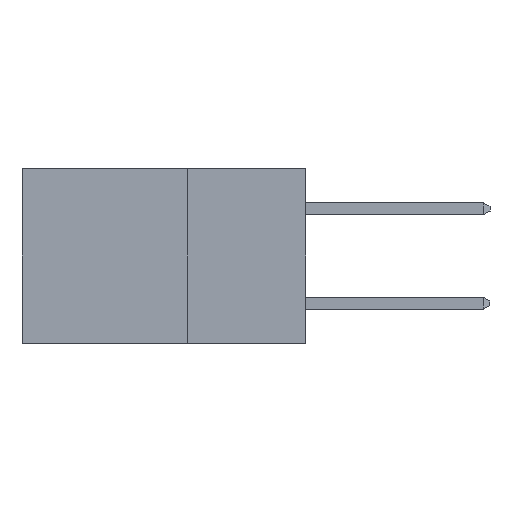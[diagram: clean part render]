
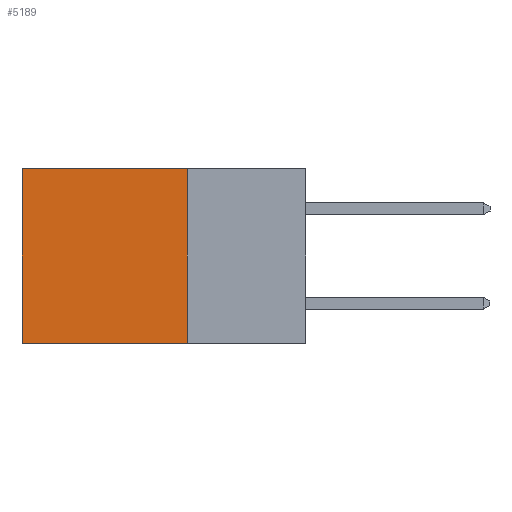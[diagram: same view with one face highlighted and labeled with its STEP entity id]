
A CAD part, left-side view. The second image highlights one B-rep face of the part: STEP entity #5189.
In plain terms, the highlighted planar face has unit normal (-1, 0, 0).
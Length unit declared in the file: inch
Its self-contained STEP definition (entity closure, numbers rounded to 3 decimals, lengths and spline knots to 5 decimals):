
#376 = ORIENTED_EDGE ( 'NONE', *, *, #2717, .T. ) ;
#1325 = ORIENTED_EDGE ( 'NONE', *, *, #2044, .T. ) ;
#2044 = EDGE_CURVE ( 'NONE', #15693, #15222, #14341, .T. ) ;
#2333 = LINE ( 'NONE', #3780, #13157 ) ;
#2617 = CARTESIAN_POINT ( 'NONE',  ( 0.298, 0.25, 0. ) ) ;
#2717 = EDGE_CURVE ( 'NONE', #15222, #8038, #10406, .T. ) ;
#2854 = VECTOR ( 'NONE', #5766, 39.37008 ) ;
#3093 = CARTESIAN_POINT ( 'NONE',  ( 0.298, 0.25, 0. ) ) ;
#3327 = VERTEX_POINT ( 'NONE', #11603 ) ;
#3507 = DIRECTION ( 'NONE',  ( 0., 1., 0. ) ) ;
#3564 = EDGE_CURVE ( 'NONE', #15693, #3327, #7947, .T. ) ;
#3630 = DIRECTION ( 'NONE',  ( 0., 0., -1. ) ) ;
#3722 = DIRECTION ( 'NONE',  ( 0., 1., 0. ) ) ;
#3780 = CARTESIAN_POINT ( 'NONE',  ( 0.298, 0.25, -0.37 ) ) ;
#3791 = CARTESIAN_POINT ( 'NONE',  ( 0.298, 0.6, -0.37 ) ) ;
#4304 = ORIENTED_EDGE ( 'NONE', *, *, #3564, .F. ) ;
#5189 = ADVANCED_FACE ( 'NONE', ( #10347 ), #5578, .F. ) ;
#5288 = CARTESIAN_POINT ( 'NONE',  ( 0.298, 0.6, 0. ) ) ;
#5578 = PLANE ( 'NONE',  #12840 ) ;
#5766 = DIRECTION ( 'NONE',  ( 0., 0., -1. ) ) ;
#7146 = CARTESIAN_POINT ( 'NONE',  ( 0.298, 0.25, 0. ) ) ;
#7499 = VECTOR ( 'NONE', #3630, 39.37008 ) ;
#7947 = LINE ( 'NONE', #14908, #7499 ) ;
#8038 = VERTEX_POINT ( 'NONE', #3791 ) ;
#9844 = DIRECTION ( 'NONE',  ( 0., 0., -1. ) ) ;
#10347 = FACE_OUTER_BOUND ( 'NONE', #12434, .T. ) ;
#10406 = LINE ( 'NONE', #5288, #2854 ) ;
#10647 = VECTOR ( 'NONE', #3507, 39.37008 ) ;
#10794 = ORIENTED_EDGE ( 'NONE', *, *, #15394, .F. ) ;
#11603 = CARTESIAN_POINT ( 'NONE',  ( 0.298, 0.25, -0.37 ) ) ;
#12434 = EDGE_LOOP ( 'NONE', ( #376, #10794, #4304, #1325 ) ) ;
#12840 = AXIS2_PLACEMENT_3D ( 'NONE', #2617, #18195, #9844 ) ;
#13157 = VECTOR ( 'NONE', #3722, 39.37008 ) ;
#14341 = LINE ( 'NONE', #3093, #10647 ) ;
#14908 = CARTESIAN_POINT ( 'NONE',  ( 0.298, 0.25, 0. ) ) ;
#15222 = VERTEX_POINT ( 'NONE', #16121 ) ;
#15394 = EDGE_CURVE ( 'NONE', #3327, #8038, #2333, .T. ) ;
#15693 = VERTEX_POINT ( 'NONE', #7146 ) ;
#16121 = CARTESIAN_POINT ( 'NONE',  ( 0.298, 0.6, 0. ) ) ;
#18195 = DIRECTION ( 'NONE',  ( 1., 0., 0. ) ) ;
